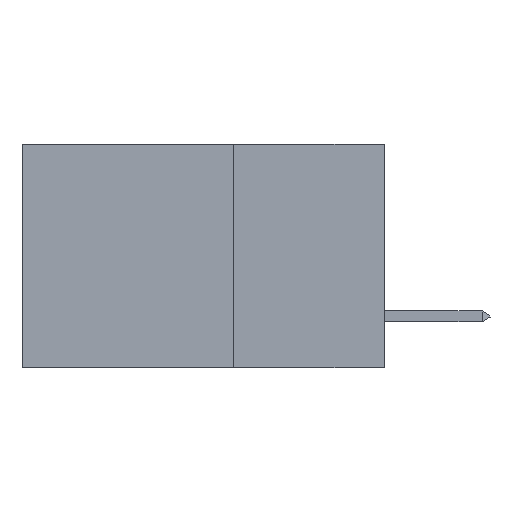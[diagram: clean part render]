
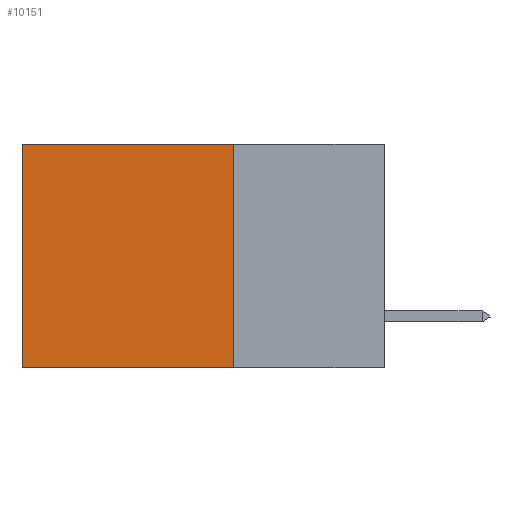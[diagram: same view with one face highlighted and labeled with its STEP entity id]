
A CAD part, left-side view. The second image highlights one B-rep face of the part: STEP entity #10151.
In plain terms, the highlighted planar face has unit normal (-1, 0, 0).
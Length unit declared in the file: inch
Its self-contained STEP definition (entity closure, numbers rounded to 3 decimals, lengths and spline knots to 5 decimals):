
#589 = EDGE_CURVE ( 'NONE', #1974, #4722, #8987, .T. ) ;
#1049 = VECTOR ( 'NONE', #2974, 39.37008 ) ;
#1428 = LINE ( 'NONE', #3208, #3455 ) ;
#1974 = VERTEX_POINT ( 'NONE', #9494 ) ;
#2974 = DIRECTION ( 'NONE',  ( 0., 1., 0. ) ) ;
#3208 = CARTESIAN_POINT ( 'NONE',  ( 0.2875, 0.25, 0. ) ) ;
#3262 = CARTESIAN_POINT ( 'NONE',  ( 0.2875, 0.25, 0. ) ) ;
#3455 = VECTOR ( 'NONE', #10265, 39.37008 ) ;
#3774 = AXIS2_PLACEMENT_3D ( 'NONE', #12255, #8252, #4974 ) ;
#4063 = PLANE ( 'NONE',  #3774 ) ;
#4313 = ORIENTED_EDGE ( 'NONE', *, *, #589, .T. ) ;
#4455 = EDGE_CURVE ( 'NONE', #1974, #5154, #1428, .T. ) ;
#4722 = VERTEX_POINT ( 'NONE', #9727 ) ;
#4828 = LINE ( 'NONE', #7214, #1049 ) ;
#4872 = LINE ( 'NONE', #12058, #8126 ) ;
#4974 = DIRECTION ( 'NONE',  ( 0., 0., -1. ) ) ;
#5154 = VERTEX_POINT ( 'NONE', #12014 ) ;
#5289 = DIRECTION ( 'NONE',  ( 0., 1., 0. ) ) ;
#5814 = EDGE_CURVE ( 'NONE', #5154, #12966, #4828, .T. ) ;
#6400 = VECTOR ( 'NONE', #5289, 39.37008 ) ;
#6754 = ORIENTED_EDGE ( 'NONE', *, *, #13039, .T. ) ;
#6993 = ORIENTED_EDGE ( 'NONE', *, *, #5814, .F. ) ;
#7022 = EDGE_LOOP ( 'NONE', ( #6754, #6993, #10377, #4313 ) ) ;
#7214 = CARTESIAN_POINT ( 'NONE',  ( 0.2875, 0.25, -0.37 ) ) ;
#7277 = FACE_OUTER_BOUND ( 'NONE', #7022, .T. ) ;
#8126 = VECTOR ( 'NONE', #11967, 39.37008 ) ;
#8252 = DIRECTION ( 'NONE',  ( 1., 0., 0. ) ) ;
#8987 = LINE ( 'NONE', #3262, #6400 ) ;
#9494 = CARTESIAN_POINT ( 'NONE',  ( 0.2875, 0.25, 0. ) ) ;
#9727 = CARTESIAN_POINT ( 'NONE',  ( 0.2875, 0.6, 0. ) ) ;
#10151 = ADVANCED_FACE ( 'NONE', ( #7277 ), #4063, .F. ) ;
#10265 = DIRECTION ( 'NONE',  ( 0., 0., -1. ) ) ;
#10377 = ORIENTED_EDGE ( 'NONE', *, *, #4455, .F. ) ;
#10597 = CARTESIAN_POINT ( 'NONE',  ( 0.2875, 0.6, -0.37 ) ) ;
#11967 = DIRECTION ( 'NONE',  ( 0., 0., -1. ) ) ;
#12014 = CARTESIAN_POINT ( 'NONE',  ( 0.2875, 0.25, -0.37 ) ) ;
#12058 = CARTESIAN_POINT ( 'NONE',  ( 0.2875, 0.6, 0. ) ) ;
#12255 = CARTESIAN_POINT ( 'NONE',  ( 0.2875, 0.25, 0. ) ) ;
#12966 = VERTEX_POINT ( 'NONE', #10597 ) ;
#13039 = EDGE_CURVE ( 'NONE', #4722, #12966, #4872, .T. ) ;
